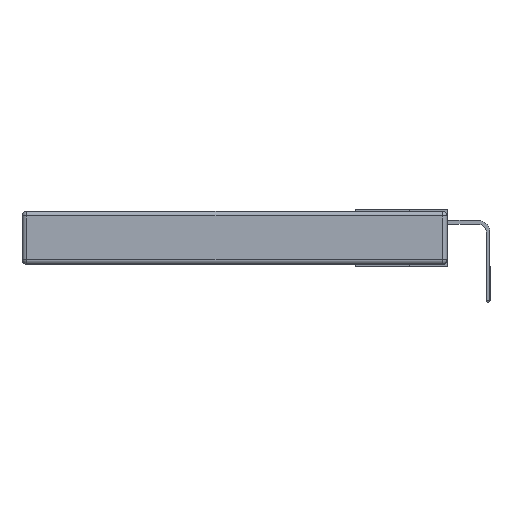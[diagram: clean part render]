
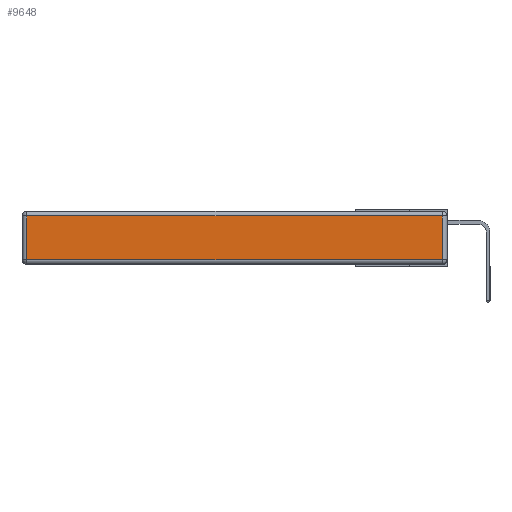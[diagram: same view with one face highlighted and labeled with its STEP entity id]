
A CAD part, left-side view. The second image highlights one B-rep face of the part: STEP entity #9648.
In plain terms, the highlighted planar face has unit normal (-1, 0, 0).
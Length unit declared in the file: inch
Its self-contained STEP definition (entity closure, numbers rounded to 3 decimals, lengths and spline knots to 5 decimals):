
#209 = ORIENTED_EDGE ( 'NONE', *, *, #15808, .T. ) ;
#2005 = DIRECTION ( 'NONE',  ( 0., 0., 1. ) ) ;
#2074 = CARTESIAN_POINT ( 'NONE',  ( 0., 0.03, -0.03 ) ) ;
#2108 = ORIENTED_EDGE ( 'NONE', *, *, #19966, .T. ) ;
#3823 = DIRECTION ( 'NONE',  ( -1., 0., 0. ) ) ;
#4889 = DIRECTION ( 'NONE',  ( 0., 1., 0. ) ) ;
#5236 = LINE ( 'NONE', #8015, #17346 ) ;
#5657 = CARTESIAN_POINT ( 'NONE',  ( 0., 0., -0.343 ) ) ;
#5896 = ORIENTED_EDGE ( 'NONE', *, *, #5919, .T. ) ;
#5919 = EDGE_CURVE ( 'NONE', #7377, #21613, #5236, .T. ) ;
#6091 = CARTESIAN_POINT ( 'NONE',  ( 0., 0., -0.313 ) ) ;
#6283 = CARTESIAN_POINT ( 'NONE',  ( 0., 2.72, -0.03 ) ) ;
#6559 = LINE ( 'NONE', #7296, #11775 ) ;
#6671 = VERTEX_POINT ( 'NONE', #19081 ) ;
#7296 = CARTESIAN_POINT ( 'NONE',  ( 0., 2.72, -0.343 ) ) ;
#7377 = VERTEX_POINT ( 'NONE', #2074 ) ;
#8015 = CARTESIAN_POINT ( 'NONE',  ( 0., 2.75, -0.03 ) ) ;
#8366 = VECTOR ( 'NONE', #2005, 39.37008 ) ;
#9648 = ADVANCED_FACE ( 'NONE', ( #19178 ), #12162, .T. ) ;
#10010 = ORIENTED_EDGE ( 'NONE', *, *, #15733, .T. ) ;
#11126 = DIRECTION ( 'NONE',  ( 0., -1., 0. ) ) ;
#11391 = VERTEX_POINT ( 'NONE', #11811 ) ;
#11775 = VECTOR ( 'NONE', #13950, 39.37008 ) ;
#11811 = CARTESIAN_POINT ( 'NONE',  ( 0., 2.72, -0.313 ) ) ;
#12162 = PLANE ( 'NONE',  #16215 ) ;
#12253 = CARTESIAN_POINT ( 'NONE',  ( 0., 0.03, -0.343 ) ) ;
#12841 = LINE ( 'NONE', #12253, #8366 ) ;
#13950 = DIRECTION ( 'NONE',  ( 0., 0., -1. ) ) ;
#14418 = VECTOR ( 'NONE', #11126, 39.37008 ) ;
#15733 = EDGE_CURVE ( 'NONE', #21613, #11391, #6559, .T. ) ;
#15808 = EDGE_CURVE ( 'NONE', #11391, #6671, #18892, .T. ) ;
#16215 = AXIS2_PLACEMENT_3D ( 'NONE', #5657, #3823, #18785 ) ;
#17346 = VECTOR ( 'NONE', #4889, 39.37008 ) ;
#18785 = DIRECTION ( 'NONE',  ( 0., 0., 1. ) ) ;
#18892 = LINE ( 'NONE', #6091, #14418 ) ;
#18916 = EDGE_LOOP ( 'NONE', ( #209, #2108, #5896, #10010 ) ) ;
#19081 = CARTESIAN_POINT ( 'NONE',  ( 0., 0.03, -0.313 ) ) ;
#19178 = FACE_OUTER_BOUND ( 'NONE', #18916, .T. ) ;
#19966 = EDGE_CURVE ( 'NONE', #6671, #7377, #12841, .T. ) ;
#21613 = VERTEX_POINT ( 'NONE', #6283 ) ;
